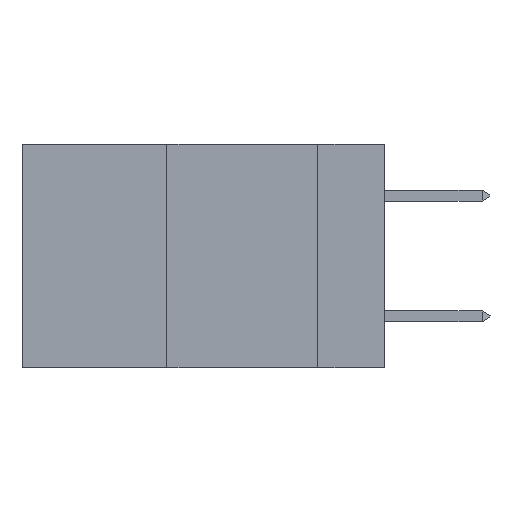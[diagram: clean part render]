
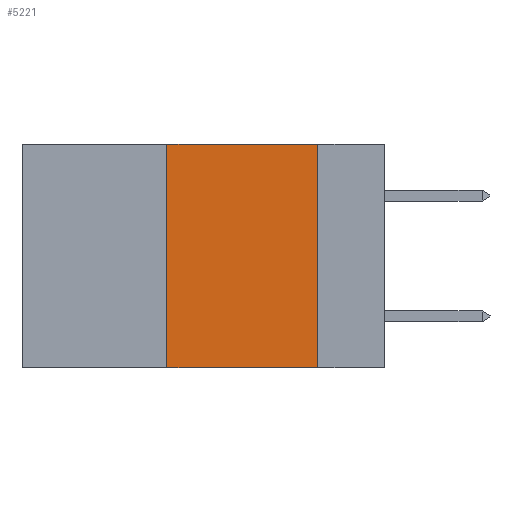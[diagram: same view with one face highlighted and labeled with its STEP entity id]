
A CAD part, left-side view. The second image highlights one B-rep face of the part: STEP entity #5221.
In plain terms, the highlighted planar face has unit normal (-1, 0, 0).
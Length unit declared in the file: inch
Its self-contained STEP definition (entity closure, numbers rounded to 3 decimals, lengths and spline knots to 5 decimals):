
#547 = FACE_OUTER_BOUND ( 'NONE', #3781, .T. ) ;
#1543 = CARTESIAN_POINT ( 'NONE',  ( 0., 0.11, -0.37 ) ) ;
#2132 = ORIENTED_EDGE ( 'NONE', *, *, #3868, .F. ) ;
#2470 = DIRECTION ( 'NONE',  ( 0., -1., 0. ) ) ;
#2956 = CARTESIAN_POINT ( 'NONE',  ( 0., 0.11, 0. ) ) ;
#3009 = CARTESIAN_POINT ( 'NONE',  ( 0., 0.6, 0. ) ) ;
#3077 = CARTESIAN_POINT ( 'NONE',  ( 0., 0.36, 0. ) ) ;
#3333 = DIRECTION ( 'NONE',  ( 1., 0., 0. ) ) ;
#3781 = EDGE_LOOP ( 'NONE', ( #26999, #14284, #2132, #17521 ) ) ;
#3868 = EDGE_CURVE ( 'NONE', #24933, #31506, #25032, .T. ) ;
#4462 = VECTOR ( 'NONE', #23137, 39.37008 ) ;
#5221 = ADVANCED_FACE ( 'NONE', ( #547 ), #23344, .F. ) ;
#5243 = LINE ( 'NONE', #22971, #21816 ) ;
#5247 = LINE ( 'NONE', #2956, #4462 ) ;
#7277 = AXIS2_PLACEMENT_3D ( 'NONE', #3009, #3333, #25604 ) ;
#7432 = CARTESIAN_POINT ( 'NONE',  ( 0., 0.11, 0. ) ) ;
#10833 = DIRECTION ( 'NONE',  ( 0., -1., 0. ) ) ;
#14284 = ORIENTED_EDGE ( 'NONE', *, *, #28929, .F. ) ;
#17088 = LINE ( 'NONE', #32140, #24424 ) ;
#17521 = ORIENTED_EDGE ( 'NONE', *, *, #29112, .T. ) ;
#18170 = CARTESIAN_POINT ( 'NONE',  ( 0., 0.36, -0.37 ) ) ;
#21816 = VECTOR ( 'NONE', #10833, 39.37008 ) ;
#22971 = CARTESIAN_POINT ( 'NONE',  ( 0., 0.6, -0.37 ) ) ;
#23137 = DIRECTION ( 'NONE',  ( 0., 0., -1. ) ) ;
#23344 = PLANE ( 'NONE',  #7277 ) ;
#23812 = CARTESIAN_POINT ( 'NONE',  ( 0., 0.36, 0. ) ) ;
#24424 = VECTOR ( 'NONE', #2470, 39.37008 ) ;
#24933 = VERTEX_POINT ( 'NONE', #18170 ) ;
#25032 = LINE ( 'NONE', #3077, #27615 ) ;
#25189 = DIRECTION ( 'NONE',  ( 0., 0., 1. ) ) ;
#25425 = VERTEX_POINT ( 'NONE', #1543 ) ;
#25604 = DIRECTION ( 'NONE',  ( 0., 0., -1. ) ) ;
#26999 = ORIENTED_EDGE ( 'NONE', *, *, #27283, .F. ) ;
#27283 = EDGE_CURVE ( 'NONE', #29846, #25425, #5247, .T. ) ;
#27615 = VECTOR ( 'NONE', #25189, 39.37008 ) ;
#28929 = EDGE_CURVE ( 'NONE', #31506, #29846, #17088, .T. ) ;
#29112 = EDGE_CURVE ( 'NONE', #24933, #25425, #5243, .T. ) ;
#29846 = VERTEX_POINT ( 'NONE', #7432 ) ;
#31506 = VERTEX_POINT ( 'NONE', #23812 ) ;
#32140 = CARTESIAN_POINT ( 'NONE',  ( 0., 0.6, 0. ) ) ;
